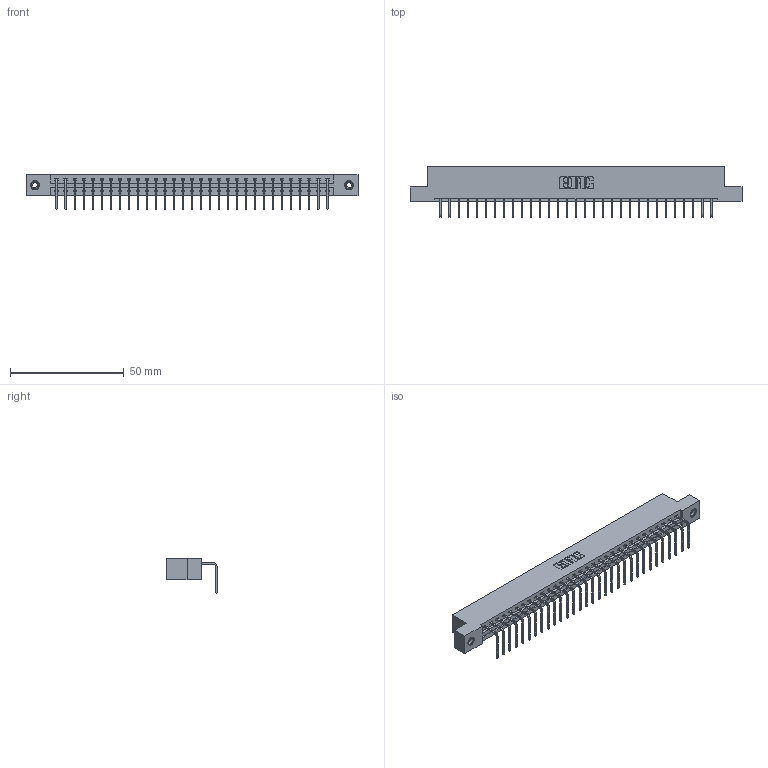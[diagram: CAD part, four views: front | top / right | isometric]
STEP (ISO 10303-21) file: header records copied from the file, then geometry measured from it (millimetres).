
FILE_DESCRIPTION (( 'STEP AP203' ), '1' );
FILE_NAME ('337-031-558-108.STEP', '2018-08-07T03:58:17', ( '' ), ( '' ), 'SwSTEP 2.0', 'SolidWorks 2016', '' );
FILE_SCHEMA (( 'CONFIG_CONTROL_DESIGN' ));
Length unit declared in the file: inch
Products named in the file (4): 337-031-558-108; 337 Part_Flush Mounting Lugs - 0.156 Dia-TI; 345-292-001_558 Tail - 2; 345-250-001_345-250-003-102
Assembly tree (34 placements, depth 2):
  337-031-558-108
    337 Part_Flush Mounting Lugs - 0.156 Dia-TI
    345-292-001_558 Tail - 2  x31
    345-250-001_345-250-003-102  x2
Bounding box: 145.85 x 22.17 x 15.37 mm (x, y, z)
Volume: 15117.4 mm3; surface area: 16224.8 mm2
Topology: 34 solids, 34 shells, 2158 faces, 6461 edges, 4258 vertices
Faces by surface type: plane 1590, cylinder 552, cone 12, torus 4
Entity records: 25736 total; most frequent: CARTESIAN_POINT 4462, ORIENTED_EDGE 4422, DIRECTION 3811, EDGE_CURVE 2211, VECTOR 2063, LINE 2063, VERTEX_POINT 1468, AXIS2_PLACEMENT_3D 874
